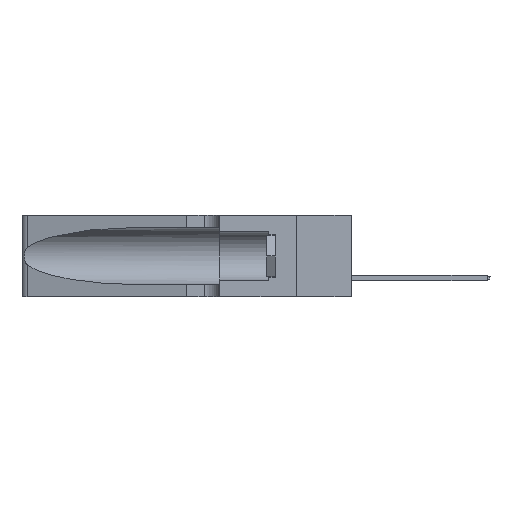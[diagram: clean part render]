
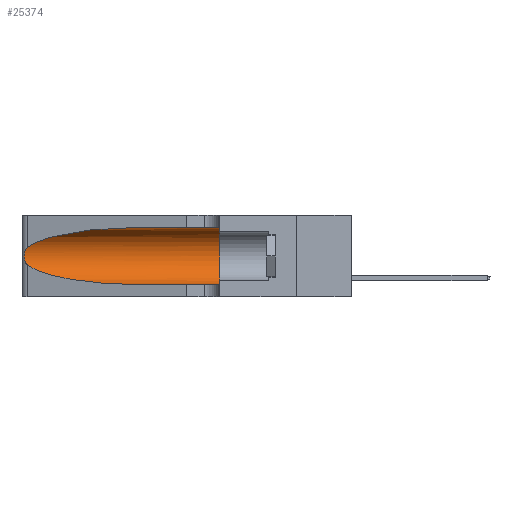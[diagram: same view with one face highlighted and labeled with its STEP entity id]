
A CAD part, left-side view. The second image highlights one B-rep face of the part: STEP entity #25374.
In plain terms, the highlighted cylindrical face has radius 3.308 mm (diameter 6.617 mm), a partial arc.
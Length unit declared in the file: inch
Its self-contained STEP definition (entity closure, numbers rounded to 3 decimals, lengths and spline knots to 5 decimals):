
#411 = DIRECTION ( 'NONE',  ( 0., 0., 1. ) ) ;
#766 = VERTEX_POINT ( 'NONE', #32712 ) ;
#869 = CARTESIAN_POINT ( 'NONE',  ( 0.1305, 0.35, 0.31525 ) ) ;
#912 = CARTESIAN_POINT ( 'NONE',  ( 0.1305, 1.61858, 0.185 ) ) ;
#1059 = CARTESIAN_POINT ( 'NONE',  ( 0.25555, 1.22993, 0.14849 ) ) ;
#1342 = CARTESIAN_POINT ( 'NONE',  ( 0.26017, 1.23833, 0.17102 ) ) ;
#1526 = LINE ( 'NONE', #31583, #30788 ) ;
#1801 = CARTESIAN_POINT ( 'NONE',  ( 0.1305, 0.72297, 0.05475 ) ) ;
#2748 = CARTESIAN_POINT ( 'NONE',  ( 0.18966, 0.96281, 0.31525 ) ) ;
#3283 = EDGE_CURVE ( 'NONE', #17988, #24535, #38616, .T. ) ;
#3766 = VERTEX_POINT ( 'NONE', #17243 ) ;
#4825 = LINE ( 'NONE', #20547, #27651 ) ;
#5151 = CIRCLE ( 'NONE', #33302, 0.13025 ) ;
#5785 = DIRECTION ( 'NONE',  ( 0., -1., 0. ) ) ;
#5864 = CARTESIAN_POINT ( 'NONE',  ( 0.2373, 1.15595, 0.28018 ) ) ;
#6477 = EDGE_CURVE ( 'NONE', #18275, #3766, #32618, .T. ) ;
#6642 = ORIENTED_EDGE ( 'NONE', *, *, #9628, .T. ) ;
#7475 = CARTESIAN_POINT ( 'NONE',  ( 0.25787, 1.23484, 0.2124 ) ) ;
#9628 = EDGE_CURVE ( 'NONE', #24535, #18275, #12418, .T. ) ;
#10869 = ORIENTED_EDGE ( 'NONE', *, *, #29079, .F. ) ;
#11654 = ORIENTED_EDGE ( 'NONE', *, *, #3283, .T. ) ;
#11726 = CARTESIAN_POINT ( 'NONE',  ( 0.1305, 0.35, 0.185 ) ) ;
#11951 = CARTESIAN_POINT ( 'NONE',  ( 0.25487, 1.22718, 0.22369 ) ) ;
#12418 = B_SPLINE_CURVE_WITH_KNOTS ( 'NONE', 3,
 ( #34150, #34013, #19229, #7475, #16354, #25547, #31374, #16492, #1342, #19094, #37423, #34548, #1059, #24995 ),
 .UNSPECIFIED., .F., .F.,
 ( 4, 2, 2, 2, 2, 2, 4 ),
 ( 0., 0.00027, 0.00053, 0.00107, 0.0016, 0.00187, 0.00214 ),
 .UNSPECIFIED. ) ;
#12962 = ORIENTED_EDGE ( 'NONE', *, *, #28723, .F. ) ;
#13087 = EDGE_LOOP ( 'NONE', ( #11654, #6642, #20871, #24125, #10869, #12962 ) ) ;
#13793 = CARTESIAN_POINT ( 'NONE',  ( 0.2373, 1.15595, 0.08982 ) ) ;
#15954 = AXIS2_PLACEMENT_3D ( 'NONE', #912, #16082, #27841 ) ;
#16082 = DIRECTION ( 'NONE',  ( 0., -1., 0. ) ) ;
#16354 = CARTESIAN_POINT ( 'NONE',  ( 0.25854, 1.2359, 0.20912 ) ) ;
#16492 = CARTESIAN_POINT ( 'NONE',  ( 0.26075, 1.23896, 0.178 ) ) ;
#17243 = CARTESIAN_POINT ( 'NONE',  ( 0.1305, 0.72297, 0.05475 ) ) ;
#17988 = VERTEX_POINT ( 'NONE', #23678 ) ;
#18275 = VERTEX_POINT ( 'NONE', #28759 ) ;
#19094 = CARTESIAN_POINT ( 'NONE',  ( 0.25856, 1.23593, 0.16098 ) ) ;
#19229 = CARTESIAN_POINT ( 'NONE',  ( 0.25639, 1.23184, 0.21858 ) ) ;
#19680 = CARTESIAN_POINT ( 'NONE',  ( 0.18966, 0.96281, 0.05475 ) ) ;
#20498 = CARTESIAN_POINT ( 'NONE',  ( 0.1305, 0.72297, 0.31525 ) ) ;
#20547 = CARTESIAN_POINT ( 'NONE',  ( 0.1305, 1.61858, 0.05475 ) ) ;
#20871 = ORIENTED_EDGE ( 'NONE', *, *, #6477, .T. ) ;
#21425 = CARTESIAN_POINT ( 'NONE',  ( 0.25487, 1.22718, 0.22369 ) ) ;
#21615 = DIRECTION ( 'NONE',  ( 0., 1., 0. ) ) ;
#22033 = VERTEX_POINT ( 'NONE', #869 ) ;
#23678 = CARTESIAN_POINT ( 'NONE',  ( 0.1305, 0.72297, 0.31525 ) ) ;
#24125 = ORIENTED_EDGE ( 'NONE', *, *, #27411, .T. ) ;
#24535 = VERTEX_POINT ( 'NONE', #21425 ) ;
#24995 = CARTESIAN_POINT ( 'NONE',  ( 0.25487, 1.22718, 0.14631 ) ) ;
#25374 = ADVANCED_FACE ( 'NONE', ( #36576 ), #28194, .F. ) ;
#25547 = CARTESIAN_POINT ( 'NONE',  ( 0.26018, 1.23835, 0.19895 ) ) ;
#27411 = EDGE_CURVE ( 'NONE', #3766, #766, #4825, .T. ) ;
#27651 = VECTOR ( 'NONE', #5785, 39.37008 ) ;
#27841 = DIRECTION ( 'NONE',  ( 0., 0., -1. ) ) ;
#28194 = CYLINDRICAL_SURFACE ( 'NONE', #15954, 0.13025 ) ;
#28723 = EDGE_CURVE ( 'NONE', #17988, #22033, #1526, .T. ) ;
#28759 = CARTESIAN_POINT ( 'NONE',  ( 0.25487, 1.22718, 0.14631 ) ) ;
#29079 = EDGE_CURVE ( 'NONE', #22033, #766, #5151, .T. ) ;
#30788 = VECTOR ( 'NONE', #31844, 39.37008 ) ;
#31374 = CARTESIAN_POINT ( 'NONE',  ( 0.26075, 1.23896, 0.19203 ) ) ;
#31583 = CARTESIAN_POINT ( 'NONE',  ( 0.1305, 1.61858, 0.31525 ) ) ;
#31844 = DIRECTION ( 'NONE',  ( 0., -1., 0. ) ) ;
#32618 =( BOUNDED_CURVE ( )  B_SPLINE_CURVE ( 3, ( #38004, #13793, #19680, #1801 ),
 .UNSPECIFIED., .F., .T. ) 
 B_SPLINE_CURVE_WITH_KNOTS ( ( 4, 4 ),
 ( 3.44316, 4.71239 ),
 .UNSPECIFIED. ) 
 CURVE ( )  GEOMETRIC_REPRESENTATION_ITEM ( )  RATIONAL_B_SPLINE_CURVE ( ( 1., 0.87, 0.87, 1. ) ) 
 REPRESENTATION_ITEM ( '' )  );
#32712 = CARTESIAN_POINT ( 'NONE',  ( 0.1305, 0.35, 0.05475 ) ) ;
#33302 = AXIS2_PLACEMENT_3D ( 'NONE', #11726, #21615, #411 ) ;
#34013 = CARTESIAN_POINT ( 'NONE',  ( 0.25555, 1.22994, 0.2215 ) ) ;
#34150 = CARTESIAN_POINT ( 'NONE',  ( 0.25487, 1.22718, 0.22369 ) ) ;
#34548 = CARTESIAN_POINT ( 'NONE',  ( 0.25639, 1.23186, 0.15144 ) ) ;
#36576 = FACE_OUTER_BOUND ( 'NONE', #13087, .T. ) ;
#37423 = CARTESIAN_POINT ( 'NONE',  ( 0.25789, 1.23486, 0.15765 ) ) ;
#38004 = CARTESIAN_POINT ( 'NONE',  ( 0.25487, 1.22718, 0.14631 ) ) ;
#38616 =( BOUNDED_CURVE ( )  B_SPLINE_CURVE ( 3, ( #20498, #2748, #5864, #11951 ),
 .UNSPECIFIED., .F., .T. ) 
 B_SPLINE_CURVE_WITH_KNOTS ( ( 4, 4 ),
 ( 1.5708, 2.84003 ),
 .UNSPECIFIED. ) 
 CURVE ( )  GEOMETRIC_REPRESENTATION_ITEM ( )  RATIONAL_B_SPLINE_CURVE ( ( 1., 0.87, 0.87, 1. ) ) 
 REPRESENTATION_ITEM ( '' )  );
